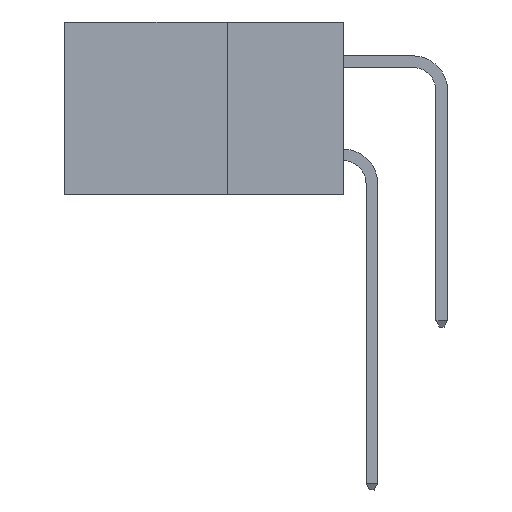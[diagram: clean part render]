
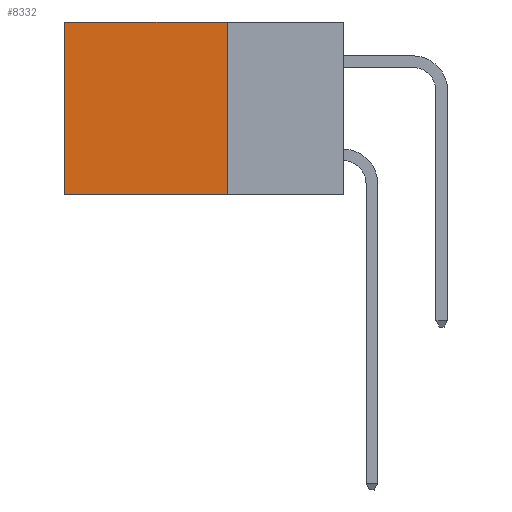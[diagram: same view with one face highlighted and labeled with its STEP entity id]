
A CAD part, left-side view. The second image highlights one B-rep face of the part: STEP entity #8332.
In plain terms, the highlighted planar face has unit normal (-1, 0, 0).
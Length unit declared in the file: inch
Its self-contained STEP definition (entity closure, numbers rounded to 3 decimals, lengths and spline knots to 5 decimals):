
#21 = DIRECTION ( 'NONE',  ( 0., 0., -1. ) ) ;
#470 = FACE_OUTER_BOUND ( 'NONE', #8072, .T. ) ;
#753 = VERTEX_POINT ( 'NONE', #7311 ) ;
#804 = ORIENTED_EDGE ( 'NONE', *, *, #3661, .T. ) ;
#960 = VECTOR ( 'NONE', #6623, 39.37008 ) ;
#1092 = LINE ( 'NONE', #12254, #10771 ) ;
#1254 = DIRECTION ( 'NONE',  ( 1., 0., 0. ) ) ;
#2739 = VERTEX_POINT ( 'NONE', #10128 ) ;
#3620 = LINE ( 'NONE', #15389, #960 ) ;
#3661 = EDGE_CURVE ( 'NONE', #10127, #2739, #1092, .T. ) ;
#3681 = EDGE_CURVE ( 'NONE', #10127, #753, #14195, .T. ) ;
#4877 = EDGE_CURVE ( 'NONE', #753, #7250, #12318, .T. ) ;
#5352 = DIRECTION ( 'NONE',  ( 0., 1., 0. ) ) ;
#5636 = VECTOR ( 'NONE', #5352, 39.37008 ) ;
#6219 = PLANE ( 'NONE',  #12186 ) ;
#6623 = DIRECTION ( 'NONE',  ( 0., 0., -1. ) ) ;
#7250 = VERTEX_POINT ( 'NONE', #12698 ) ;
#7311 = CARTESIAN_POINT ( 'NONE',  ( 0.298, 0.25, -0.37 ) ) ;
#7823 = ORIENTED_EDGE ( 'NONE', *, *, #3681, .F. ) ;
#8031 = ORIENTED_EDGE ( 'NONE', *, *, #4877, .F. ) ;
#8072 = EDGE_LOOP ( 'NONE', ( #10527, #8031, #7823, #804 ) ) ;
#8332 = ADVANCED_FACE ( 'NONE', ( #470 ), #6219, .F. ) ;
#8461 = CARTESIAN_POINT ( 'NONE',  ( 0.298, 0.25, 0. ) ) ;
#8611 = CARTESIAN_POINT ( 'NONE',  ( 0.298, 0.25, 0. ) ) ;
#10127 = VERTEX_POINT ( 'NONE', #15122 ) ;
#10128 = CARTESIAN_POINT ( 'NONE',  ( 0.298, 0.6, 0. ) ) ;
#10527 = ORIENTED_EDGE ( 'NONE', *, *, #12338, .T. ) ;
#10771 = VECTOR ( 'NONE', #11621, 39.37008 ) ;
#11073 = CARTESIAN_POINT ( 'NONE',  ( 0.298, 0.25, -0.37 ) ) ;
#11411 = DIRECTION ( 'NONE',  ( 0., 0., -1. ) ) ;
#11621 = DIRECTION ( 'NONE',  ( 0., 1., 0. ) ) ;
#12186 = AXIS2_PLACEMENT_3D ( 'NONE', #8461, #1254, #21 ) ;
#12254 = CARTESIAN_POINT ( 'NONE',  ( 0.298, 0.25, 0. ) ) ;
#12318 = LINE ( 'NONE', #11073, #5636 ) ;
#12338 = EDGE_CURVE ( 'NONE', #2739, #7250, #3620, .T. ) ;
#12698 = CARTESIAN_POINT ( 'NONE',  ( 0.298, 0.6, -0.37 ) ) ;
#13802 = VECTOR ( 'NONE', #11411, 39.37008 ) ;
#14195 = LINE ( 'NONE', #8611, #13802 ) ;
#15122 = CARTESIAN_POINT ( 'NONE',  ( 0.298, 0.25, 0. ) ) ;
#15389 = CARTESIAN_POINT ( 'NONE',  ( 0.298, 0.6, 0. ) ) ;
